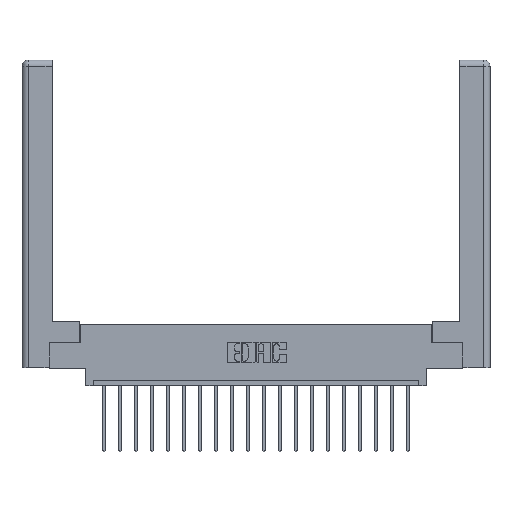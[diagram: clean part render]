
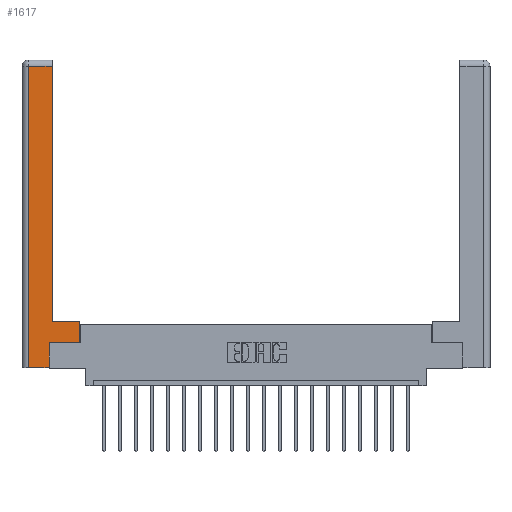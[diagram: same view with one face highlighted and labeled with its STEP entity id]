
A CAD part, top view. The second image highlights one B-rep face of the part: STEP entity #1617.
In plain terms, the highlighted planar face has unit normal (0, 0, 1).
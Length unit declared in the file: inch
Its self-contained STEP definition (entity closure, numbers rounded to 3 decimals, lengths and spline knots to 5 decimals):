
#26 = CARTESIAN_POINT ( 'NONE',  ( 0.265, 0., 0. ) ) ;
#51 = CARTESIAN_POINT ( 'NONE',  ( 0.265, 0.245, 0. ) ) ;
#263 = ORIENTED_EDGE ( 'NONE', *, *, #4352, .T. ) ;
#265 = VECTOR ( 'NONE', #13982, 39.37008 ) ;
#362 = ORIENTED_EDGE ( 'NONE', *, *, #19636, .T. ) ;
#812 = LINE ( 'NONE', #3921, #15707 ) ;
#1617 = ADVANCED_FACE ( 'NONE', ( #3906 ), #15563, .F. ) ;
#1698 = LINE ( 'NONE', #51, #18047 ) ;
#2985 = LINE ( 'NONE', #3351, #12400 ) ;
#3260 = CARTESIAN_POINT ( 'NONE',  ( 0.565, 0.245, 0. ) ) ;
#3351 = CARTESIAN_POINT ( 'NONE',  ( 0.565, 0.245, 0. ) ) ;
#3906 = FACE_OUTER_BOUND ( 'NONE', #7615, .T. ) ;
#3921 = CARTESIAN_POINT ( 'NONE',  ( 0.295, 3., 0. ) ) ;
#3983 = CARTESIAN_POINT ( 'NONE',  ( 0.0615, 0., 0. ) ) ;
#4352 = EDGE_CURVE ( 'NONE', #5113, #11242, #13764, .T. ) ;
#4881 = CARTESIAN_POINT ( 'NONE',  ( 0.565, 0.45, 0. ) ) ;
#5113 = VERTEX_POINT ( 'NONE', #15385 ) ;
#6039 = ORIENTED_EDGE ( 'NONE', *, *, #9258, .T. ) ;
#6062 = DIRECTION ( 'NONE',  ( 0., 0., -1. ) ) ;
#6930 = ORIENTED_EDGE ( 'NONE', *, *, #19641, .T. ) ;
#7232 = CARTESIAN_POINT ( 'NONE',  ( 0.0615, 0., 0. ) ) ;
#7615 = EDGE_LOOP ( 'NONE', ( #6039, #263, #362, #10850, #19377, #18307, #6930, #10145 ) ) ;
#8692 = LINE ( 'NONE', #3983, #18130 ) ;
#9258 = EDGE_CURVE ( 'NONE', #11953, #5113, #812, .T. ) ;
#9458 = VERTEX_POINT ( 'NONE', #16807 ) ;
#9783 = DIRECTION ( 'NONE',  ( -1., 0., 0. ) ) ;
#10145 = ORIENTED_EDGE ( 'NONE', *, *, #13028, .T. ) ;
#10527 = DIRECTION ( 'NONE',  ( 0., -1., 0. ) ) ;
#10727 = VERTEX_POINT ( 'NONE', #3260 ) ;
#10850 = ORIENTED_EDGE ( 'NONE', *, *, #19917, .T. ) ;
#11052 = VERTEX_POINT ( 'NONE', #7232 ) ;
#11242 = VERTEX_POINT ( 'NONE', #19007 ) ;
#11953 = VERTEX_POINT ( 'NONE', #16567 ) ;
#12100 = CARTESIAN_POINT ( 'NONE',  ( 0.565, 0.45, 0. ) ) ;
#12400 = VECTOR ( 'NONE', #12850, 39.37008 ) ;
#12432 = VERTEX_POINT ( 'NONE', #4881 ) ;
#12477 = EDGE_CURVE ( 'NONE', #18567, #9458, #1698, .T. ) ;
#12686 = LINE ( 'NONE', #26, #265 ) ;
#12850 = DIRECTION ( 'NONE',  ( 1., 0., 0. ) ) ;
#12851 = CARTESIAN_POINT ( 'NONE',  ( 0.295, 0.45, 0. ) ) ;
#12890 = AXIS2_PLACEMENT_3D ( 'NONE', #18585, #6062, #17137 ) ;
#13028 = EDGE_CURVE ( 'NONE', #12432, #11953, #18509, .T. ) ;
#13688 = VECTOR ( 'NONE', #15308, 39.37008 ) ;
#13764 = LINE ( 'NONE', #20394, #14270 ) ;
#13982 = DIRECTION ( 'NONE',  ( 1., 0., 0. ) ) ;
#14007 = EDGE_CURVE ( 'NONE', #9458, #10727, #2985, .T. ) ;
#14270 = VECTOR ( 'NONE', #20254, 39.37008 ) ;
#14334 = VECTOR ( 'NONE', #9783, 39.37008 ) ;
#14874 = DIRECTION ( 'NONE',  ( 0., 1., 0. ) ) ;
#15308 = DIRECTION ( 'NONE',  ( 0., 1., 0. ) ) ;
#15385 = CARTESIAN_POINT ( 'NONE',  ( 0.295, 2.94, 0. ) ) ;
#15563 = PLANE ( 'NONE',  #12890 ) ;
#15707 = VECTOR ( 'NONE', #16522, 39.37008 ) ;
#16345 = CARTESIAN_POINT ( 'NONE',  ( 0.265, 0., 0. ) ) ;
#16522 = DIRECTION ( 'NONE',  ( 0., 1., 0. ) ) ;
#16567 = CARTESIAN_POINT ( 'NONE',  ( 0.295, 0.45, 0. ) ) ;
#16641 = LINE ( 'NONE', #12100, #13688 ) ;
#16807 = CARTESIAN_POINT ( 'NONE',  ( 0.265, 0.245, 0. ) ) ;
#17137 = DIRECTION ( 'NONE',  ( -1., 0., 0. ) ) ;
#18047 = VECTOR ( 'NONE', #14874, 39.37008 ) ;
#18130 = VECTOR ( 'NONE', #10527, 39.37008 ) ;
#18307 = ORIENTED_EDGE ( 'NONE', *, *, #14007, .T. ) ;
#18509 = LINE ( 'NONE', #12851, #14334 ) ;
#18567 = VERTEX_POINT ( 'NONE', #16345 ) ;
#18585 = CARTESIAN_POINT ( 'NONE',  ( 0., 0., 0. ) ) ;
#19007 = CARTESIAN_POINT ( 'NONE',  ( 0.0615, 2.94, 0. ) ) ;
#19377 = ORIENTED_EDGE ( 'NONE', *, *, #12477, .T. ) ;
#19636 = EDGE_CURVE ( 'NONE', #11242, #11052, #8692, .T. ) ;
#19641 = EDGE_CURVE ( 'NONE', #10727, #12432, #16641, .T. ) ;
#19917 = EDGE_CURVE ( 'NONE', #11052, #18567, #12686, .T. ) ;
#20254 = DIRECTION ( 'NONE',  ( -1., 0., 0. ) ) ;
#20394 = CARTESIAN_POINT ( 'NONE',  ( 0.0615, 2.94, 0. ) ) ;
